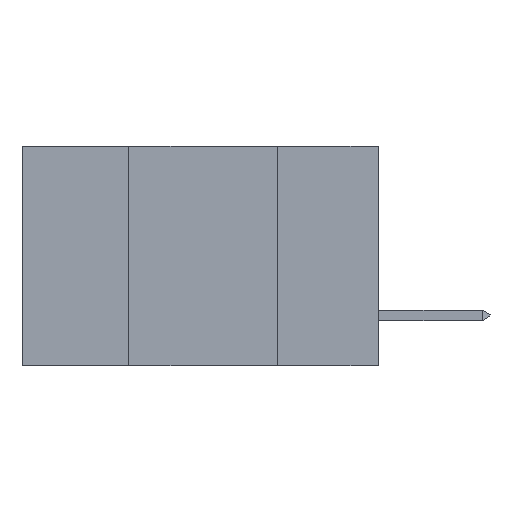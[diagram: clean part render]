
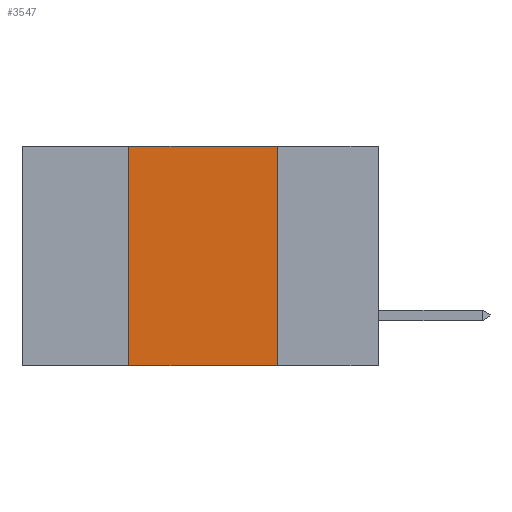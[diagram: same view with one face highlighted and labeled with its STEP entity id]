
A CAD part, left-side view. The second image highlights one B-rep face of the part: STEP entity #3547.
In plain terms, the highlighted planar face has unit normal (-1, 0, 0).
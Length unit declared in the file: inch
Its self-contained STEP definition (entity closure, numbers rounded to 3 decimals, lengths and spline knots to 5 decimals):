
#91 = CARTESIAN_POINT ( 'NONE',  ( 0., 0.17, 0. ) ) ;
#220 = PLANE ( 'NONE',  #845 ) ;
#837 = VECTOR ( 'NONE', #15902, 39.37008 ) ;
#845 = AXIS2_PLACEMENT_3D ( 'NONE', #10097, #1807, #20355 ) ;
#1366 = CARTESIAN_POINT ( 'NONE',  ( 0., 0.17, 0. ) ) ;
#1622 = CARTESIAN_POINT ( 'NONE',  ( 0., 0.17, -0.37 ) ) ;
#1807 = DIRECTION ( 'NONE',  ( 1., 0., 0. ) ) ;
#2734 = EDGE_CURVE ( 'NONE', #17976, #8295, #18071, .T. ) ;
#3047 = DIRECTION ( 'NONE',  ( 0., 0., -1. ) ) ;
#3547 = ADVANCED_FACE ( 'NONE', ( #18176 ), #220, .F. ) ;
#5013 = CARTESIAN_POINT ( 'NONE',  ( 0., 0.6, 0. ) ) ;
#5049 = EDGE_LOOP ( 'NONE', ( #9049, #14345, #9658, #15988 ) ) ;
#5822 = VERTEX_POINT ( 'NONE', #91 ) ;
#6895 = EDGE_CURVE ( 'NONE', #13926, #5822, #17897, .T. ) ;
#7473 = VECTOR ( 'NONE', #18179, 39.37008 ) ;
#8295 = VERTEX_POINT ( 'NONE', #1622 ) ;
#9049 = ORIENTED_EDGE ( 'NONE', *, *, #19507, .F. ) ;
#9625 = LINE ( 'NONE', #1366, #20584 ) ;
#9658 = ORIENTED_EDGE ( 'NONE', *, *, #17477, .F. ) ;
#10097 = CARTESIAN_POINT ( 'NONE',  ( 0., 0.6, 0. ) ) ;
#11021 = VECTOR ( 'NONE', #20361, 39.37008 ) ;
#12468 = CARTESIAN_POINT ( 'NONE',  ( 0., 0.6, -0.37 ) ) ;
#12548 = CARTESIAN_POINT ( 'NONE',  ( 0., 0.42, 0. ) ) ;
#13926 = VERTEX_POINT ( 'NONE', #12548 ) ;
#14345 = ORIENTED_EDGE ( 'NONE', *, *, #6895, .F. ) ;
#15902 = DIRECTION ( 'NONE',  ( 0., -1., 0. ) ) ;
#15988 = ORIENTED_EDGE ( 'NONE', *, *, #2734, .T. ) ;
#17477 = EDGE_CURVE ( 'NONE', #17976, #13926, #19865, .T. ) ;
#17785 = CARTESIAN_POINT ( 'NONE',  ( 0., 0.42, -0.37 ) ) ;
#17897 = LINE ( 'NONE', #5013, #7473 ) ;
#17976 = VERTEX_POINT ( 'NONE', #17785 ) ;
#18071 = LINE ( 'NONE', #12468, #837 ) ;
#18176 = FACE_OUTER_BOUND ( 'NONE', #5049, .T. ) ;
#18179 = DIRECTION ( 'NONE',  ( 0., -1., 0. ) ) ;
#18686 = CARTESIAN_POINT ( 'NONE',  ( 0., 0.42, 0. ) ) ;
#19507 = EDGE_CURVE ( 'NONE', #5822, #8295, #9625, .T. ) ;
#19865 = LINE ( 'NONE', #18686, #11021 ) ;
#20355 = DIRECTION ( 'NONE',  ( 0., 0., -1. ) ) ;
#20361 = DIRECTION ( 'NONE',  ( 0., 0., 1. ) ) ;
#20584 = VECTOR ( 'NONE', #3047, 39.37008 ) ;
